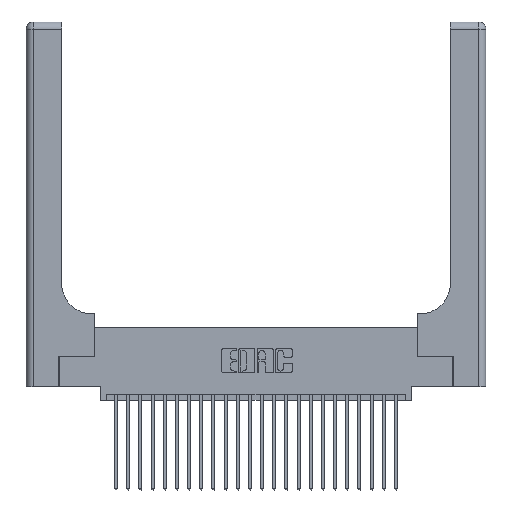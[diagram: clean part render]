
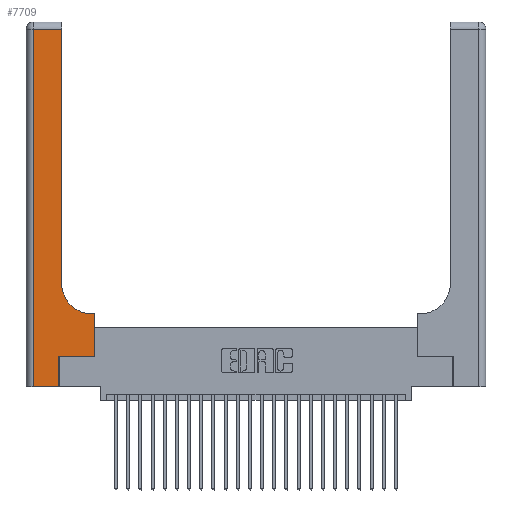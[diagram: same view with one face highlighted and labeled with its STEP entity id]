
A CAD part, top view. The second image highlights one B-rep face of the part: STEP entity #7709.
In plain terms, the highlighted planar face has unit normal (0, 0, 1).
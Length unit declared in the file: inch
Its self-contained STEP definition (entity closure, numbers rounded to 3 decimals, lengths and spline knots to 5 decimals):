
#1698 = ORIENTED_EDGE ( 'NONE', *, *, #9372, .T. ) ;
#2125 = DIRECTION ( 'NONE',  ( 0., 0., -1. ) ) ;
#2479 = CARTESIAN_POINT ( 'NONE',  ( 0.2915, 0.6, 0.37 ) ) ;
#2691 = VERTEX_POINT ( 'NONE', #25416 ) ;
#3026 = EDGE_CURVE ( 'NONE', #25343, #20988, #19059, .T. ) ;
#3104 = PLANE ( 'NONE',  #4587 ) ;
#3201 = VECTOR ( 'NONE', #21660, 39.37008 ) ;
#3345 = CARTESIAN_POINT ( 'NONE',  ( 0.06, 3., 0.37 ) ) ;
#3544 = CARTESIAN_POINT ( 'NONE',  ( 0.269, 0.25, 0.37 ) ) ;
#3759 = CIRCLE ( 'NONE', #5367, 0.25 ) ;
#3986 = ORIENTED_EDGE ( 'NONE', *, *, #3026, .T. ) ;
#4587 = AXIS2_PLACEMENT_3D ( 'NONE', #17620, #5271, #19648 ) ;
#4882 = LINE ( 'NONE', #23553, #15215 ) ;
#5150 = VECTOR ( 'NONE', #12813, 39.37008 ) ;
#5271 = DIRECTION ( 'NONE',  ( 0., 0., -1. ) ) ;
#5336 = EDGE_CURVE ( 'NONE', #10441, #16578, #3759, .T. ) ;
#5367 = AXIS2_PLACEMENT_3D ( 'NONE', #14527, #2125, #16586 ) ;
#5471 = FACE_OUTER_BOUND ( 'NONE', #19509, .T. ) ;
#5647 = DIRECTION ( 'NONE',  ( 0., 1., 0. ) ) ;
#6218 = DIRECTION ( 'NONE',  ( 1., 0., 0. ) ) ;
#6901 = ORIENTED_EDGE ( 'NONE', *, *, #17406, .T. ) ;
#7244 = CARTESIAN_POINT ( 'NONE',  ( 0.5585, 0.25, 0.37 ) ) ;
#7577 = VERTEX_POINT ( 'NONE', #15856 ) ;
#7709 = ADVANCED_FACE ( 'NONE', ( #5471 ), #3104, .F. ) ;
#7753 = ORIENTED_EDGE ( 'NONE', *, *, #9987, .T. ) ;
#8683 = CARTESIAN_POINT ( 'NONE',  ( 0.2915, 0.85, 0.37 ) ) ;
#9372 = EDGE_CURVE ( 'NONE', #2691, #16844, #18706, .T. ) ;
#9431 = EDGE_CURVE ( 'NONE', #26309, #18209, #26329, .T. ) ;
#9789 = DIRECTION ( 'NONE',  ( 1., 0., 0. ) ) ;
#9987 = EDGE_CURVE ( 'NONE', #20988, #26309, #13559, .T. ) ;
#10441 = VERTEX_POINT ( 'NONE', #19227 ) ;
#10770 = CARTESIAN_POINT ( 'NONE',  ( 0.269, 0., 0.37 ) ) ;
#11211 = EDGE_CURVE ( 'NONE', #16844, #25343, #24022, .T. ) ;
#11297 = DIRECTION ( 'NONE',  ( 0., 1., 0. ) ) ;
#11628 = ORIENTED_EDGE ( 'NONE', *, *, #20113, .T. ) ;
#11824 = ORIENTED_EDGE ( 'NONE', *, *, #5336, .T. ) ;
#12446 = CARTESIAN_POINT ( 'NONE',  ( 0.269, 0.25, 0.37 ) ) ;
#12813 = DIRECTION ( 'NONE',  ( -1., 0., 0. ) ) ;
#13559 = LINE ( 'NONE', #19600, #3201 ) ;
#13629 = VECTOR ( 'NONE', #6218, 39.37008 ) ;
#13672 = CARTESIAN_POINT ( 'NONE',  ( 0., 2.94, 0.37 ) ) ;
#14527 = CARTESIAN_POINT ( 'NONE',  ( 0.5415, 0.85, 0.37 ) ) ;
#15215 = VECTOR ( 'NONE', #11297, 39.37008 ) ;
#15856 = CARTESIAN_POINT ( 'NONE',  ( 0.5585, 0.6, 0.37 ) ) ;
#15933 = CARTESIAN_POINT ( 'NONE',  ( 0.5585, 0.25, 0.37 ) ) ;
#16578 = VERTEX_POINT ( 'NONE', #8683 ) ;
#16586 = DIRECTION ( 'NONE',  ( 1., 0., 0. ) ) ;
#16711 = EDGE_CURVE ( 'NONE', #16578, #2691, #4882, .T. ) ;
#16844 = VERTEX_POINT ( 'NONE', #19258 ) ;
#17406 = EDGE_CURVE ( 'NONE', #7577, #10441, #20925, .T. ) ;
#17620 = CARTESIAN_POINT ( 'NONE',  ( 0., 3., 0.37 ) ) ;
#17771 = DIRECTION ( 'NONE',  ( -1., 0., 0. ) ) ;
#17966 = VECTOR ( 'NONE', #19800, 39.37008 ) ;
#18192 = ORIENTED_EDGE ( 'NONE', *, *, #9431, .T. ) ;
#18209 = VERTEX_POINT ( 'NONE', #7244 ) ;
#18543 = CARTESIAN_POINT ( 'NONE',  ( 0., 0., 0.37 ) ) ;
#18706 = LINE ( 'NONE', #13672, #22209 ) ;
#18788 = ORIENTED_EDGE ( 'NONE', *, *, #16711, .T. ) ;
#19008 = CARTESIAN_POINT ( 'NONE',  ( 0.06, 0., 0.37 ) ) ;
#19059 = LINE ( 'NONE', #18543, #13629 ) ;
#19227 = CARTESIAN_POINT ( 'NONE',  ( 0.5415, 0.6, 0.37 ) ) ;
#19258 = CARTESIAN_POINT ( 'NONE',  ( 0.06, 2.94, 0.37 ) ) ;
#19409 = VECTOR ( 'NONE', #5647, 39.37008 ) ;
#19509 = EDGE_LOOP ( 'NONE', ( #18788, #1698, #21233, #3986, #7753, #18192, #11628, #6901, #11824 ) ) ;
#19600 = CARTESIAN_POINT ( 'NONE',  ( 0.269, 0., 0.37 ) ) ;
#19648 = DIRECTION ( 'NONE',  ( -1., 0., 0. ) ) ;
#19800 = DIRECTION ( 'NONE',  ( 0., -1., 0. ) ) ;
#20065 = LINE ( 'NONE', #15933, #19409 ) ;
#20113 = EDGE_CURVE ( 'NONE', #18209, #7577, #20065, .T. ) ;
#20925 = LINE ( 'NONE', #2479, #5150 ) ;
#20988 = VERTEX_POINT ( 'NONE', #10770 ) ;
#21233 = ORIENTED_EDGE ( 'NONE', *, *, #11211, .T. ) ;
#21660 = DIRECTION ( 'NONE',  ( 0., 1., 0. ) ) ;
#22209 = VECTOR ( 'NONE', #17771, 39.37008 ) ;
#23553 = CARTESIAN_POINT ( 'NONE',  ( 0.2915, 3., 0.37 ) ) ;
#24022 = LINE ( 'NONE', #3345, #17966 ) ;
#25343 = VERTEX_POINT ( 'NONE', #19008 ) ;
#25416 = CARTESIAN_POINT ( 'NONE',  ( 0.2915, 2.94, 0.37 ) ) ;
#25707 = VECTOR ( 'NONE', #9789, 39.37008 ) ;
#26309 = VERTEX_POINT ( 'NONE', #12446 ) ;
#26329 = LINE ( 'NONE', #3544, #25707 ) ;
